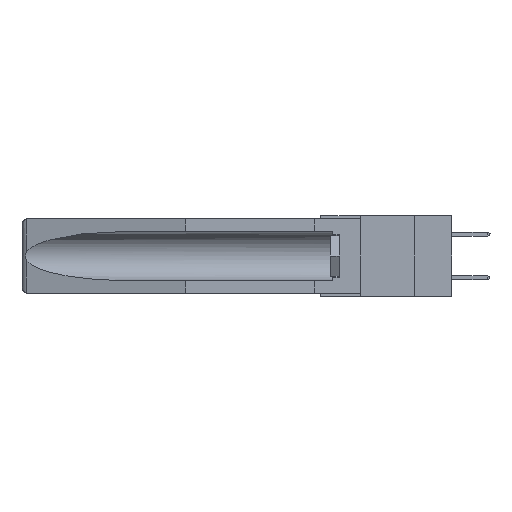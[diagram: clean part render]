
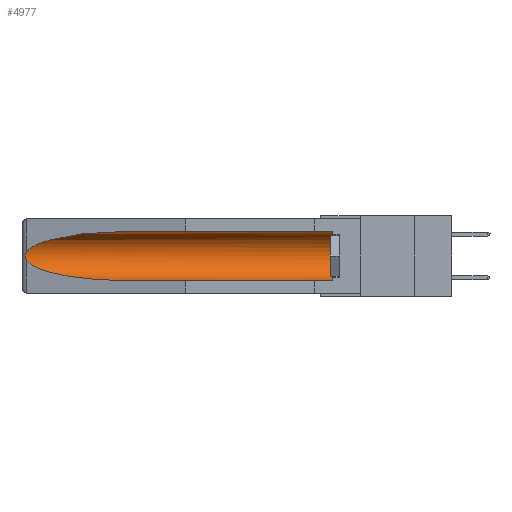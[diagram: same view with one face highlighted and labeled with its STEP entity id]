
A CAD part, left-side view. The second image highlights one B-rep face of the part: STEP entity #4977.
In plain terms, the highlighted cylindrical face has radius 2.857 mm (diameter 5.715 mm), a partial arc.
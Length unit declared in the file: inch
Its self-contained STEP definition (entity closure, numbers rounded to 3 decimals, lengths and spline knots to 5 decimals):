
#43 = CYLINDRICAL_SURFACE ( 'NONE', #19437, 0.1125 ) ;
#1732 = DIRECTION ( 'NONE',  ( 0., 0., 1. ) ) ;
#2039 = CARTESIAN_POINT ( 'NONE',  ( 0.155, 1.07973, -0.284 ) ) ;
#2493 = DIRECTION ( 'NONE',  ( 0., 1., 0. ) ) ;
#2818 = CARTESIAN_POINT ( 'NONE',  ( 0.25451, 1.48313, -0.09465 ) ) ;
#3049 = CARTESIAN_POINT ( 'NONE',  ( 0.155, 0.126, -0.059 ) ) ;
#3850 = CARTESIAN_POINT ( 'NONE',  ( 0.155, 1.07973, -0.284 ) ) ;
#3905 = CARTESIAN_POINT ( 'NONE',  ( 0.155, 1.07973, -0.059 ) ) ;
#3932 = ORIENTED_EDGE ( 'NONE', *, *, #12143, .T. ) ;
#4765 = DIRECTION ( 'NONE',  ( 0., -1., 0. ) ) ;
#4977 = ADVANCED_FACE ( 'NONE', ( #6962 ), #43, .F. ) ;
#4994 = CARTESIAN_POINT ( 'NONE',  ( 0.2675, 1.53308, -0.17534 ) ) ;
#5368 = CARTESIAN_POINT ( 'NONE',  ( 0.26537, 1.52718, -0.19328 ) ) ;
#6285 = CARTESIAN_POINT ( 'NONE',  ( 0.26537, 1.52718, -0.14972 ) ) ;
#6327 = VERTEX_POINT ( 'NONE', #5368 ) ;
#6424 = CARTESIAN_POINT ( 'NONE',  ( 0.155, -0.30754, -0.284 ) ) ;
#6651 = CIRCLE ( 'NONE', #22911, 0.1125 ) ;
#6847 = CARTESIAN_POINT ( 'NONE',  ( 0.26597, 1.52961, -0.15275 ) ) ;
#6962 = FACE_OUTER_BOUND ( 'NONE', #7238, .T. ) ;
#7090 = VECTOR ( 'NONE', #13729, 39.37008 ) ;
#7238 = EDGE_LOOP ( 'NONE', ( #24795, #3932, #21999, #23673, #22732, #19253 ) ) ;
#7494 = CARTESIAN_POINT ( 'NONE',  ( 0.21114, 1.30732, -0.284 ) ) ;
#8142 = VERTEX_POINT ( 'NONE', #3850 ) ;
#8247 = EDGE_CURVE ( 'NONE', #20259, #8142, #22776, .T. ) ;
#8598 = LINE ( 'NONE', #17404, #7090 ) ;
#8721 = EDGE_CURVE ( 'NONE', #13863, #17526, #8598, .T. ) ;
#8831 = VERTEX_POINT ( 'NONE', #6285 ) ;
#8952 =( BOUNDED_CURVE ( )  B_SPLINE_CURVE ( 3, ( #19242, #24816, #7494, #2039 ),
 .UNSPECIFIED., .F., .F. ) 
 B_SPLINE_CURVE_WITH_KNOTS ( ( 4, 4 ),
 ( 0.1948, 1.5708 ),
 .UNSPECIFIED. ) 
 CURVE ( )  GEOMETRIC_REPRESENTATION_ITEM ( )  RATIONAL_B_SPLINE_CURVE ( ( 1., 0.848, 0.848, 1. ) ) 
 REPRESENTATION_ITEM ( '' )  );
#9156 = CARTESIAN_POINT ( 'NONE',  ( 0.26655, 1.53094, -0.18657 ) ) ;
#10070 = CARTESIAN_POINT ( 'NONE',  ( 0.26537, 1.52718, -0.14972 ) ) ;
#11137 = CARTESIAN_POINT ( 'NONE',  ( 0.155, 0.126, -0.284 ) ) ;
#12143 = EDGE_CURVE ( 'NONE', #8831, #6327, #19370, .T. ) ;
#12679 = CARTESIAN_POINT ( 'NONE',  ( 0.2673, 1.53269, -0.17917 ) ) ;
#12759 = CARTESIAN_POINT ( 'NONE',  ( 0.2673, 1.5327, -0.16383 ) ) ;
#13729 = DIRECTION ( 'NONE',  ( 0., 1., 0. ) ) ;
#13863 = VERTEX_POINT ( 'NONE', #3049 ) ;
#14177 =( BOUNDED_CURVE ( )  B_SPLINE_CURVE ( 3, ( #19597, #22047, #2818, #10070 ),
 .UNSPECIFIED., .F., .F. ) 
 B_SPLINE_CURVE_WITH_KNOTS ( ( 4, 4 ),
 ( 4.71239, 6.08839 ),
 .UNSPECIFIED. ) 
 CURVE ( )  GEOMETRIC_REPRESENTATION_ITEM ( )  RATIONAL_B_SPLINE_CURVE ( ( 1., 0.848, 0.848, 1. ) ) 
 REPRESENTATION_ITEM ( '' )  );
#14590 = CARTESIAN_POINT ( 'NONE',  ( 0.155, -0.30754, -0.1715 ) ) ;
#14776 = CARTESIAN_POINT ( 'NONE',  ( 0.2675, 1.53308, -0.16763 ) ) ;
#15261 = VECTOR ( 'NONE', #2493, 39.37008 ) ;
#16300 = EDGE_CURVE ( 'NONE', #20259, #13863, #6651, .T. ) ;
#16768 = CARTESIAN_POINT ( 'NONE',  ( 0.26537, 1.52718, -0.14972 ) ) ;
#17404 = CARTESIAN_POINT ( 'NONE',  ( 0.155, -0.30754, -0.059 ) ) ;
#17526 = VERTEX_POINT ( 'NONE', #3905 ) ;
#18188 = DIRECTION ( 'NONE',  ( 0., 0., 1. ) ) ;
#18433 = CARTESIAN_POINT ( 'NONE',  ( 0.26654, 1.53092, -0.15636 ) ) ;
#19028 = EDGE_CURVE ( 'NONE', #6327, #8142, #8952, .T. ) ;
#19242 = CARTESIAN_POINT ( 'NONE',  ( 0.26537, 1.52718, -0.19328 ) ) ;
#19253 = ORIENTED_EDGE ( 'NONE', *, *, #8721, .T. ) ;
#19370 = B_SPLINE_CURVE_WITH_KNOTS ( 'NONE', 3,
 ( #16768, #6847, #18433, #12759, #14776, #4994, #12679, #9156, #22565, #20554 ),
 .UNSPECIFIED., .F., .F.,
 ( 4, 2, 2, 2, 4 ),
 ( 0., 0.00029, 0.00058, 0.00087, 0.00117 ),
 .UNSPECIFIED. ) ;
#19437 = AXIS2_PLACEMENT_3D ( 'NONE', #14590, #22564, #1732 ) ;
#19597 = CARTESIAN_POINT ( 'NONE',  ( 0.155, 1.07973, -0.059 ) ) ;
#20259 = VERTEX_POINT ( 'NONE', #11137 ) ;
#20472 = CARTESIAN_POINT ( 'NONE',  ( 0.155, 0.126, -0.1715 ) ) ;
#20554 = CARTESIAN_POINT ( 'NONE',  ( 0.26537, 1.52718, -0.19328 ) ) ;
#21999 = ORIENTED_EDGE ( 'NONE', *, *, #19028, .T. ) ;
#22047 = CARTESIAN_POINT ( 'NONE',  ( 0.21114, 1.30732, -0.059 ) ) ;
#22056 = EDGE_CURVE ( 'NONE', #17526, #8831, #14177, .T. ) ;
#22564 = DIRECTION ( 'NONE',  ( 0., 1., 0. ) ) ;
#22565 = CARTESIAN_POINT ( 'NONE',  ( 0.26597, 1.5296, -0.19026 ) ) ;
#22732 = ORIENTED_EDGE ( 'NONE', *, *, #16300, .T. ) ;
#22776 = LINE ( 'NONE', #6424, #15261 ) ;
#22911 = AXIS2_PLACEMENT_3D ( 'NONE', #20472, #4765, #18188 ) ;
#23673 = ORIENTED_EDGE ( 'NONE', *, *, #8247, .F. ) ;
#24795 = ORIENTED_EDGE ( 'NONE', *, *, #22056, .T. ) ;
#24816 = CARTESIAN_POINT ( 'NONE',  ( 0.25451, 1.48313, -0.24835 ) ) ;
